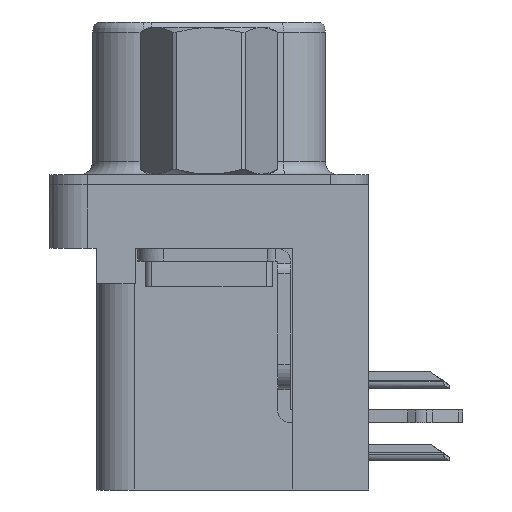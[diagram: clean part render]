
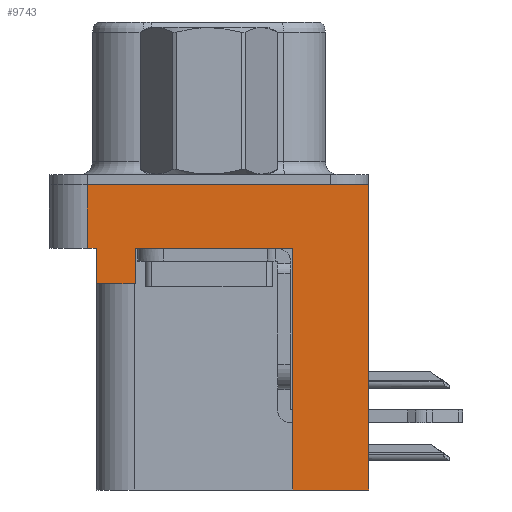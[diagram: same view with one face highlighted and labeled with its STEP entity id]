
A CAD part, left-side view. The second image highlights one B-rep face of the part: STEP entity #9743.
In plain terms, the highlighted planar face has unit normal (-1, 0, 0).
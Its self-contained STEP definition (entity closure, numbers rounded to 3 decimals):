
#397 = FACE_OUTER_BOUND ( 'NONE', #24900, .T. ) ;
#616 = VECTOR ( 'NONE', #20015, 1000. ) ;
#864 = EDGE_CURVE ( 'NONE', #15657, #20290, #6339, .T. ) ;
#1310 = VERTEX_POINT ( 'NONE', #2148 ) ;
#1843 = DIRECTION ( 'NONE',  ( 0., 0., 1. ) ) ;
#1900 = VECTOR ( 'NONE', #1843, 1000. ) ;
#2148 = CARTESIAN_POINT ( 'NONE',  ( -3., 4.425, -2.5 ) ) ;
#2453 = CARTESIAN_POINT ( 'NONE',  ( -3., 2.895, -3.9 ) ) ;
#2615 = CARTESIAN_POINT ( 'NONE',  ( -3., 4.425, -3.9 ) ) ;
#3053 = VERTEX_POINT ( 'NONE', #26257 ) ;
#4047 = CARTESIAN_POINT ( 'NONE',  ( -3., 4.775, -2.5 ) ) ;
#4464 = VECTOR ( 'NONE', #19214, 1000. ) ;
#4597 = DIRECTION ( 'NONE',  ( 0., 0., 1. ) ) ;
#5145 = ORIENTED_EDGE ( 'NONE', *, *, #7317, .T. ) ;
#5185 = ORIENTED_EDGE ( 'NONE', *, *, #26685, .T. ) ;
#5670 = CARTESIAN_POINT ( 'NONE',  ( -3., -6.275, -2.5 ) ) ;
#6092 = CARTESIAN_POINT ( 'NONE',  ( -3., -6.275, -2.5 ) ) ;
#6339 = LINE ( 'NONE', #4047, #1900 ) ;
#7053 = DIRECTION ( 'NONE',  ( -1., 0., 0. ) ) ;
#7117 = CARTESIAN_POINT ( 'NONE',  ( -3., 4.425, -3.9 ) ) ;
#7317 = EDGE_CURVE ( 'NONE', #25433, #20123, #7673, .T. ) ;
#7643 = LINE ( 'NONE', #8521, #17133 ) ;
#7673 = LINE ( 'NONE', #5670, #24986 ) ;
#8373 = EDGE_CURVE ( 'NONE', #8387, #20123, #27316, .T. ) ;
#8387 = VERTEX_POINT ( 'NONE', #14764 ) ;
#8521 = CARTESIAN_POINT ( 'NONE',  ( -3., 2.895, -3.9 ) ) ;
#8724 = VERTEX_POINT ( 'NONE', #22956 ) ;
#9109 = DIRECTION ( 'NONE',  ( 0., -1., 0. ) ) ;
#9732 = EDGE_CURVE ( 'NONE', #3053, #23506, #26526, .T. ) ;
#9743 = ADVANCED_FACE ( 'NONE', ( #397 ), #11145, .T. ) ;
#10120 = EDGE_CURVE ( 'NONE', #8724, #1310, #21151, .T. ) ;
#10234 = LINE ( 'NONE', #16951, #4464 ) ;
#11145 = PLANE ( 'NONE',  #24787 ) ;
#11281 = VERTEX_POINT ( 'NONE', #2453 ) ;
#11486 = ORIENTED_EDGE ( 'NONE', *, *, #24920, .F. ) ;
#12380 = VECTOR ( 'NONE', #27653, 1000. ) ;
#12557 = CARTESIAN_POINT ( 'NONE',  ( -3., -3.295, -12. ) ) ;
#13332 = LINE ( 'NONE', #23733, #14386 ) ;
#13513 = ORIENTED_EDGE ( 'NONE', *, *, #18927, .F. ) ;
#13635 = ORIENTED_EDGE ( 'NONE', *, *, #9732, .T. ) ;
#13687 = DIRECTION ( 'NONE',  ( 0., 0., 1. ) ) ;
#14386 = VECTOR ( 'NONE', #25892, 1000. ) ;
#14764 = CARTESIAN_POINT ( 'NONE',  ( -3., -3.295, -12. ) ) ;
#15657 = VERTEX_POINT ( 'NONE', #21292 ) ;
#15840 = DIRECTION ( 'NONE',  ( 0., -1., 0. ) ) ;
#16951 = CARTESIAN_POINT ( 'NONE',  ( -3., -6.275, -2.5 ) ) ;
#17133 = VECTOR ( 'NONE', #23687, 1000. ) ;
#18913 = ORIENTED_EDGE ( 'NONE', *, *, #8373, .F. ) ;
#18927 = EDGE_CURVE ( 'NONE', #11281, #8724, #18933, .T. ) ;
#18933 = LINE ( 'NONE', #7117, #616 ) ;
#19097 = VECTOR ( 'NONE', #13687, 1000. ) ;
#19214 = DIRECTION ( 'NONE',  ( 0., -1., 0. ) ) ;
#19274 = CARTESIAN_POINT ( 'NONE',  ( -3., -6.275, -2.5 ) ) ;
#20015 = DIRECTION ( 'NONE',  ( 0., 1., 0. ) ) ;
#20123 = VERTEX_POINT ( 'NONE', #24703 ) ;
#20280 = EDGE_CURVE ( 'NONE', #11281, #25433, #7643, .T. ) ;
#20290 = VERTEX_POINT ( 'NONE', #21532 ) ;
#20646 = ORIENTED_EDGE ( 'NONE', *, *, #20870, .F. ) ;
#20870 = EDGE_CURVE ( 'NONE', #3053, #8387, #13332, .T. ) ;
#21151 = LINE ( 'NONE', #2615, #19097 ) ;
#21292 = CARTESIAN_POINT ( 'NONE',  ( -3., 4.775, -2.5 ) ) ;
#21532 = CARTESIAN_POINT ( 'NONE',  ( -3., 4.775, 0. ) ) ;
#22855 = VECTOR ( 'NONE', #4597, 1000. ) ;
#22956 = CARTESIAN_POINT ( 'NONE',  ( -3., 4.425, -3.9 ) ) ;
#23506 = VERTEX_POINT ( 'NONE', #26246 ) ;
#23687 = DIRECTION ( 'NONE',  ( 0., 0., 1. ) ) ;
#23733 = CARTESIAN_POINT ( 'NONE',  ( -3., -3.295, -12. ) ) ;
#23911 = ORIENTED_EDGE ( 'NONE', *, *, #20280, .T. ) ;
#24220 = DIRECTION ( 'NONE',  ( 0., 0., 1. ) ) ;
#24703 = CARTESIAN_POINT ( 'NONE',  ( -3., -3.295, -2.5 ) ) ;
#24787 = AXIS2_PLACEMENT_3D ( 'NONE', #6092, #7053, #24220 ) ;
#24900 = EDGE_LOOP ( 'NONE', ( #11486, #25356, #5185, #25362, #13513, #23911, #5145, #18913, #20646, #13635 ) ) ;
#24920 = EDGE_CURVE ( 'NONE', #20290, #23506, #27037, .T. ) ;
#24986 = VECTOR ( 'NONE', #15840, 1000. ) ;
#25356 = ORIENTED_EDGE ( 'NONE', *, *, #864, .F. ) ;
#25362 = ORIENTED_EDGE ( 'NONE', *, *, #10120, .F. ) ;
#25433 = VERTEX_POINT ( 'NONE', #25662 ) ;
#25662 = CARTESIAN_POINT ( 'NONE',  ( -3., 2.895, -2.5 ) ) ;
#25892 = DIRECTION ( 'NONE',  ( 0., 1., 0. ) ) ;
#26246 = CARTESIAN_POINT ( 'NONE',  ( -3., -6.275, 0. ) ) ;
#26257 = CARTESIAN_POINT ( 'NONE',  ( -3., -6.275, -12. ) ) ;
#26337 = VECTOR ( 'NONE', #9109, 1000. ) ;
#26360 = CARTESIAN_POINT ( 'NONE',  ( -3., -6.275, 0. ) ) ;
#26526 = LINE ( 'NONE', #19274, #22855 ) ;
#26685 = EDGE_CURVE ( 'NONE', #15657, #1310, #10234, .T. ) ;
#27037 = LINE ( 'NONE', #26360, #26337 ) ;
#27316 = LINE ( 'NONE', #12557, #12380 ) ;
#27653 = DIRECTION ( 'NONE',  ( 0., 0., 1. ) ) ;
